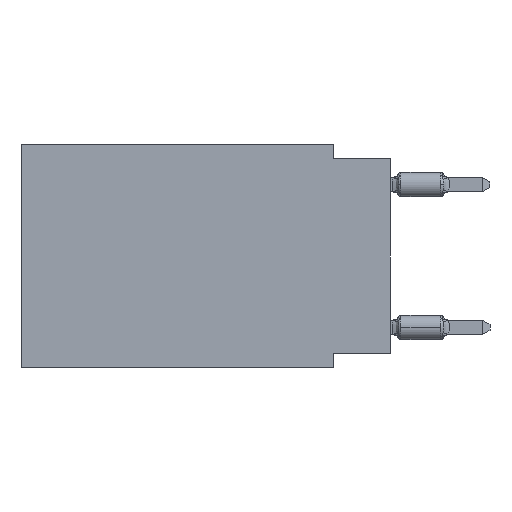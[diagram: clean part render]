
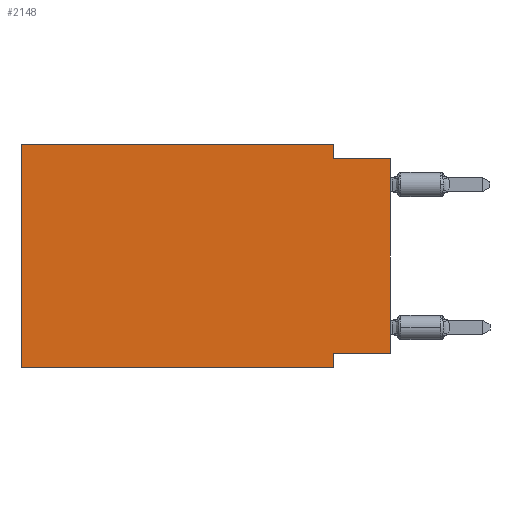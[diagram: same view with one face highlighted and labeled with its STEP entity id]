
A CAD part, left-side view. The second image highlights one B-rep face of the part: STEP entity #2148.
In plain terms, the highlighted planar face has unit normal (-1, 0, 0).
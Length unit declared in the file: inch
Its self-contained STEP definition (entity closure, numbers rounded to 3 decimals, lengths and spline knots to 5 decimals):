
#1285 = ORIENTED_EDGE ( 'NONE', *, *, #3458, .F. ) ;
#2025 = VECTOR ( 'NONE', #43565, 39.37008 ) ;
#2148 = ADVANCED_FACE ( 'NONE', ( #15344 ), #4698, .F. ) ;
#2281 = VECTOR ( 'NONE', #33705, 39.37008 ) ;
#3238 = CARTESIAN_POINT ( 'NONE',  ( 0., 0.1, -0.365 ) ) ;
#3458 = EDGE_CURVE ( 'NONE', #20298, #41925, #38396, .T. ) ;
#3932 = VERTEX_POINT ( 'NONE', #28688 ) ;
#4034 = LINE ( 'NONE', #41684, #25484 ) ;
#4455 = CARTESIAN_POINT ( 'NONE',  ( 0., 0.645, -0.39 ) ) ;
#4651 = VERTEX_POINT ( 'NONE', #12500 ) ;
#4698 = PLANE ( 'NONE',  #37115 ) ;
#5209 = CARTESIAN_POINT ( 'NONE',  ( 0., 0.645, 0. ) ) ;
#5252 = ORIENTED_EDGE ( 'NONE', *, *, #43698, .T. ) ;
#5575 = DIRECTION ( 'NONE',  ( 1., 0., 0. ) ) ;
#7358 = CARTESIAN_POINT ( 'NONE',  ( 0., 0.1, -0.39 ) ) ;
#7476 = ORIENTED_EDGE ( 'NONE', *, *, #40334, .F. ) ;
#8129 = CARTESIAN_POINT ( 'NONE',  ( 0., 0.1, -0.025 ) ) ;
#8276 = VECTOR ( 'NONE', #21798, 39.37008 ) ;
#9005 = EDGE_CURVE ( 'NONE', #25859, #15119, #27962, .T. ) ;
#9684 = EDGE_CURVE ( 'NONE', #3932, #25859, #31607, .T. ) ;
#10732 = LINE ( 'NONE', #30579, #2281 ) ;
#10927 = EDGE_CURVE ( 'NONE', #3932, #4651, #10732, .T. ) ;
#12500 = CARTESIAN_POINT ( 'NONE',  ( 0., 0., -0.025 ) ) ;
#12813 = LINE ( 'NONE', #4455, #8276 ) ;
#13246 = CARTESIAN_POINT ( 'NONE',  ( 0., 0., -0.025 ) ) ;
#14553 = EDGE_CURVE ( 'NONE', #38823, #4651, #43782, .T. ) ;
#15119 = VERTEX_POINT ( 'NONE', #7358 ) ;
#15344 = FACE_OUTER_BOUND ( 'NONE', #19732, .T. ) ;
#16561 = VECTOR ( 'NONE', #19782, 39.37008 ) ;
#16876 = LINE ( 'NONE', #27551, #16561 ) ;
#17932 = CARTESIAN_POINT ( 'NONE',  ( 0., 0.1, -0.39 ) ) ;
#17999 = CARTESIAN_POINT ( 'NONE',  ( 0., 0.645, 0. ) ) ;
#18249 = DIRECTION ( 'NONE',  ( 0., 0., -1. ) ) ;
#18760 = DIRECTION ( 'NONE',  ( 0., 0., 1. ) ) ;
#19732 = EDGE_LOOP ( 'NONE', ( #39088, #40839, #7476, #28183, #1285, #5252, #42811, #34218 ) ) ;
#19782 = DIRECTION ( 'NONE',  ( 0., -1., 0. ) ) ;
#19860 = CARTESIAN_POINT ( 'NONE',  ( 0., 0., -0.365 ) ) ;
#20298 = VERTEX_POINT ( 'NONE', #27833 ) ;
#20488 = VERTEX_POINT ( 'NONE', #23542 ) ;
#21798 = DIRECTION ( 'NONE',  ( 0., -1., 0. ) ) ;
#21849 = EDGE_CURVE ( 'NONE', #41925, #20488, #16876, .T. ) ;
#23542 = CARTESIAN_POINT ( 'NONE',  ( 0., 0.1, 0. ) ) ;
#24936 = CARTESIAN_POINT ( 'NONE',  ( 0., 0.645, 0. ) ) ;
#25484 = VECTOR ( 'NONE', #42123, 39.37008 ) ;
#25859 = VERTEX_POINT ( 'NONE', #3238 ) ;
#27551 = CARTESIAN_POINT ( 'NONE',  ( 0., 0.645, 0. ) ) ;
#27833 = CARTESIAN_POINT ( 'NONE',  ( 0., 0.645, -0.39 ) ) ;
#27962 = LINE ( 'NONE', #17932, #42121 ) ;
#28183 = ORIENTED_EDGE ( 'NONE', *, *, #21849, .F. ) ;
#28688 = CARTESIAN_POINT ( 'NONE',  ( 0., 0., -0.365 ) ) ;
#29831 = VECTOR ( 'NONE', #30135, 39.37008 ) ;
#30135 = DIRECTION ( 'NONE',  ( 0., 1., 0. ) ) ;
#30579 = CARTESIAN_POINT ( 'NONE',  ( 0., 0., 0. ) ) ;
#31545 = DIRECTION ( 'NONE',  ( 0., 0., -1. ) ) ;
#31607 = LINE ( 'NONE', #19860, #29831 ) ;
#33705 = DIRECTION ( 'NONE',  ( 0., 0., 1. ) ) ;
#34218 = ORIENTED_EDGE ( 'NONE', *, *, #9684, .F. ) ;
#36517 = VECTOR ( 'NONE', #18760, 39.37008 ) ;
#37115 = AXIS2_PLACEMENT_3D ( 'NONE', #24936, #5575, #18249 ) ;
#38396 = LINE ( 'NONE', #5209, #36517 ) ;
#38823 = VERTEX_POINT ( 'NONE', #8129 ) ;
#39088 = ORIENTED_EDGE ( 'NONE', *, *, #10927, .T. ) ;
#40334 = EDGE_CURVE ( 'NONE', #20488, #38823, #4034, .T. ) ;
#40839 = ORIENTED_EDGE ( 'NONE', *, *, #14553, .F. ) ;
#41684 = CARTESIAN_POINT ( 'NONE',  ( 0., 0.1, 0. ) ) ;
#41925 = VERTEX_POINT ( 'NONE', #17999 ) ;
#42121 = VECTOR ( 'NONE', #31545, 39.37008 ) ;
#42123 = DIRECTION ( 'NONE',  ( 0., 0., -1. ) ) ;
#42811 = ORIENTED_EDGE ( 'NONE', *, *, #9005, .F. ) ;
#43565 = DIRECTION ( 'NONE',  ( 0., -1., 0. ) ) ;
#43698 = EDGE_CURVE ( 'NONE', #20298, #15119, #12813, .T. ) ;
#43782 = LINE ( 'NONE', #13246, #2025 ) ;
